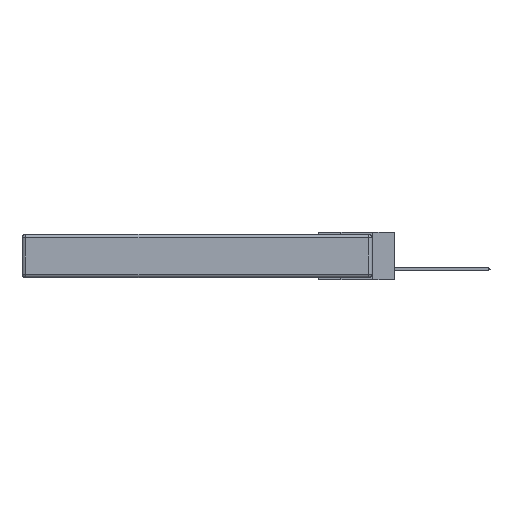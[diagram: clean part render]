
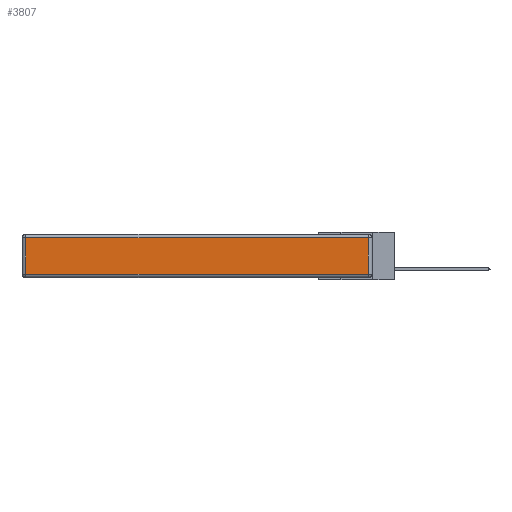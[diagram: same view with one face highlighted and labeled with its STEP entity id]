
A CAD part, left-side view. The second image highlights one B-rep face of the part: STEP entity #3807.
In plain terms, the highlighted planar face has unit normal (-1, 0, 0).
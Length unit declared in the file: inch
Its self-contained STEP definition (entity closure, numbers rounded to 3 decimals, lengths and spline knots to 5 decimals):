
#258 = VECTOR ( 'NONE', #9091, 39.37008 ) ;
#1593 = ORIENTED_EDGE ( 'NONE', *, *, #3947, .T. ) ;
#1905 = EDGE_CURVE ( 'NONE', #12264, #14882, #2120, .T. ) ;
#2076 = LINE ( 'NONE', #13356, #4422 ) ;
#2120 = LINE ( 'NONE', #15042, #258 ) ;
#3288 = LINE ( 'NONE', #16584, #13260 ) ;
#3807 = ADVANCED_FACE ( 'NONE', ( #7670 ), #14590, .T. ) ;
#3947 = EDGE_CURVE ( 'NONE', #9623, #4898, #2076, .T. ) ;
#4119 = CARTESIAN_POINT ( 'NONE',  ( 0., 0.03, -0.03 ) ) ;
#4301 = AXIS2_PLACEMENT_3D ( 'NONE', #5725, #16061, #8468 ) ;
#4422 = VECTOR ( 'NONE', #17819, 39.37008 ) ;
#4440 = EDGE_CURVE ( 'NONE', #4898, #12264, #7408, .T. ) ;
#4898 = VERTEX_POINT ( 'NONE', #4119 ) ;
#5110 = ORIENTED_EDGE ( 'NONE', *, *, #1905, .T. ) ;
#5725 = CARTESIAN_POINT ( 'NONE',  ( 0., 0., -0.343 ) ) ;
#5769 = VECTOR ( 'NONE', #11381, 39.37008 ) ;
#7408 = LINE ( 'NONE', #9768, #5769 ) ;
#7670 = FACE_OUTER_BOUND ( 'NONE', #9447, .T. ) ;
#8468 = DIRECTION ( 'NONE',  ( 0., 0., 1. ) ) ;
#9091 = DIRECTION ( 'NONE',  ( 0., 0., -1. ) ) ;
#9316 = DIRECTION ( 'NONE',  ( 0., -1., 0. ) ) ;
#9447 = EDGE_LOOP ( 'NONE', ( #14753, #1593, #18361, #5110 ) ) ;
#9623 = VERTEX_POINT ( 'NONE', #16978 ) ;
#9768 = CARTESIAN_POINT ( 'NONE',  ( 0., 2.75, -0.03 ) ) ;
#10251 = CARTESIAN_POINT ( 'NONE',  ( 0., 2.72, -0.313 ) ) ;
#11381 = DIRECTION ( 'NONE',  ( 0., 1., 0. ) ) ;
#12264 = VERTEX_POINT ( 'NONE', #15665 ) ;
#13260 = VECTOR ( 'NONE', #9316, 39.37008 ) ;
#13356 = CARTESIAN_POINT ( 'NONE',  ( 0., 0.03, -0.343 ) ) ;
#14590 = PLANE ( 'NONE',  #4301 ) ;
#14753 = ORIENTED_EDGE ( 'NONE', *, *, #18445, .T. ) ;
#14882 = VERTEX_POINT ( 'NONE', #10251 ) ;
#15042 = CARTESIAN_POINT ( 'NONE',  ( 0., 2.72, -0.343 ) ) ;
#15665 = CARTESIAN_POINT ( 'NONE',  ( 0., 2.72, -0.03 ) ) ;
#16061 = DIRECTION ( 'NONE',  ( -1., 0., 0. ) ) ;
#16584 = CARTESIAN_POINT ( 'NONE',  ( 0., 0., -0.313 ) ) ;
#16978 = CARTESIAN_POINT ( 'NONE',  ( 0., 0.03, -0.313 ) ) ;
#17819 = DIRECTION ( 'NONE',  ( 0., 0., 1. ) ) ;
#18361 = ORIENTED_EDGE ( 'NONE', *, *, #4440, .T. ) ;
#18445 = EDGE_CURVE ( 'NONE', #14882, #9623, #3288, .T. ) ;
